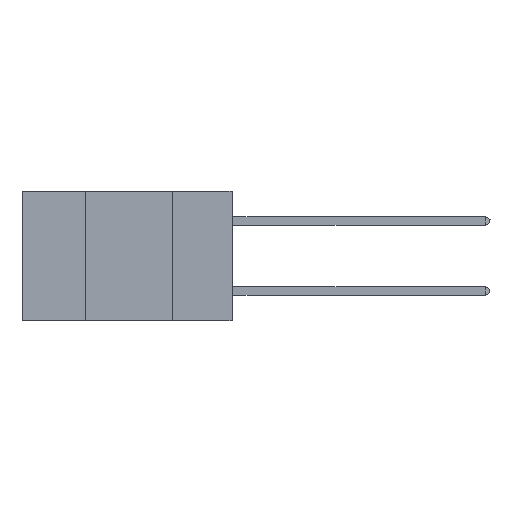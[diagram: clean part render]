
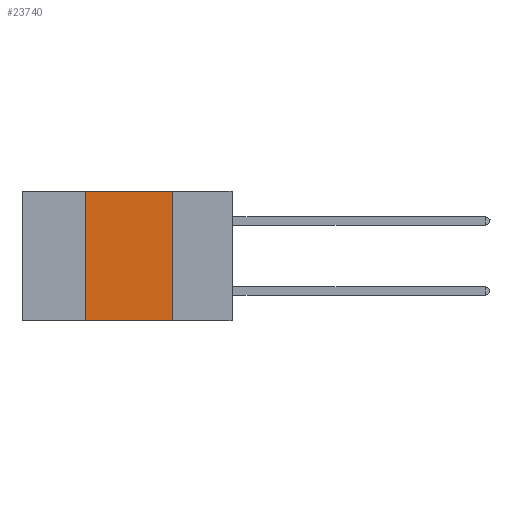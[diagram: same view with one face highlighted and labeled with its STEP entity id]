
A CAD part, left-side view. The second image highlights one B-rep face of the part: STEP entity #23740.
In plain terms, the highlighted planar face has unit normal (-1, 0, 0).
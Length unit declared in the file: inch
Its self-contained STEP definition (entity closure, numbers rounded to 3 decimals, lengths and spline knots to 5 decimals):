
#573 = VECTOR ( 'NONE', #5437, 39.37008 ) ;
#1550 = VERTEX_POINT ( 'NONE', #17981 ) ;
#1623 = CARTESIAN_POINT ( 'NONE',  ( 0., 0.17, 0. ) ) ;
#2048 = DIRECTION ( 'NONE',  ( 0., 0., -1. ) ) ;
#3616 = CARTESIAN_POINT ( 'NONE',  ( 0., 0.42, -0.37 ) ) ;
#4097 = CARTESIAN_POINT ( 'NONE',  ( 0., 0.6, 0. ) ) ;
#5437 = DIRECTION ( 'NONE',  ( 0., 0., -1. ) ) ;
#5973 = FACE_OUTER_BOUND ( 'NONE', #20920, .T. ) ;
#6087 = EDGE_CURVE ( 'NONE', #16145, #22044, #17986, .T. ) ;
#7519 = ORIENTED_EDGE ( 'NONE', *, *, #9069, .F. ) ;
#7611 = ORIENTED_EDGE ( 'NONE', *, *, #6087, .T. ) ;
#7705 = PLANE ( 'NONE',  #18550 ) ;
#8457 = VECTOR ( 'NONE', #15754, 39.37008 ) ;
#9069 = EDGE_CURVE ( 'NONE', #16145, #12996, #12789, .T. ) ;
#9765 = DIRECTION ( 'NONE',  ( 1., 0., 0. ) ) ;
#10500 = VECTOR ( 'NONE', #20510, 39.37008 ) ;
#11912 = CARTESIAN_POINT ( 'NONE',  ( 0., 0.42, 0. ) ) ;
#12222 = CARTESIAN_POINT ( 'NONE',  ( 0., 0.17, -0.37 ) ) ;
#12789 = LINE ( 'NONE', #13017, #10500 ) ;
#12996 = VERTEX_POINT ( 'NONE', #11912 ) ;
#13017 = CARTESIAN_POINT ( 'NONE',  ( 0., 0.42, 0. ) ) ;
#15320 = EDGE_CURVE ( 'NONE', #1550, #22044, #18451, .T. ) ;
#15754 = DIRECTION ( 'NONE',  ( 0., -1., 0. ) ) ;
#16145 = VERTEX_POINT ( 'NONE', #3616 ) ;
#16221 = EDGE_CURVE ( 'NONE', #12996, #1550, #18944, .T. ) ;
#16548 = ORIENTED_EDGE ( 'NONE', *, *, #15320, .F. ) ;
#17005 = VECTOR ( 'NONE', #18224, 39.37008 ) ;
#17297 = ORIENTED_EDGE ( 'NONE', *, *, #16221, .F. ) ;
#17981 = CARTESIAN_POINT ( 'NONE',  ( 0., 0.17, 0. ) ) ;
#17986 = LINE ( 'NONE', #21880, #17005 ) ;
#18224 = DIRECTION ( 'NONE',  ( 0., -1., 0. ) ) ;
#18451 = LINE ( 'NONE', #1623, #573 ) ;
#18550 = AXIS2_PLACEMENT_3D ( 'NONE', #20940, #9765, #2048 ) ;
#18944 = LINE ( 'NONE', #4097, #8457 ) ;
#20510 = DIRECTION ( 'NONE',  ( 0., 0., 1. ) ) ;
#20920 = EDGE_LOOP ( 'NONE', ( #16548, #17297, #7519, #7611 ) ) ;
#20940 = CARTESIAN_POINT ( 'NONE',  ( 0., 0.6, 0. ) ) ;
#21880 = CARTESIAN_POINT ( 'NONE',  ( 0., 0.6, -0.37 ) ) ;
#22044 = VERTEX_POINT ( 'NONE', #12222 ) ;
#23740 = ADVANCED_FACE ( 'NONE', ( #5973 ), #7705, .F. ) ;
